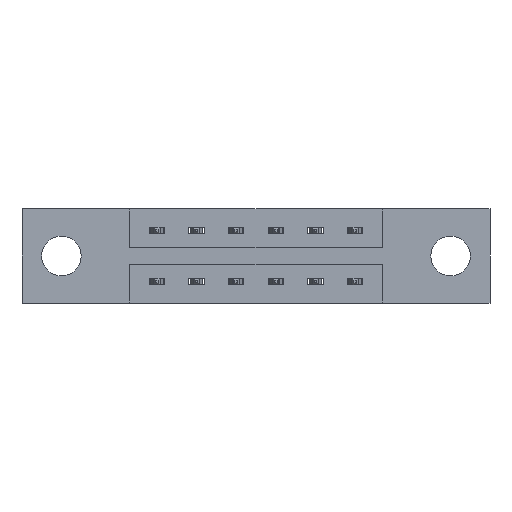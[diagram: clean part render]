
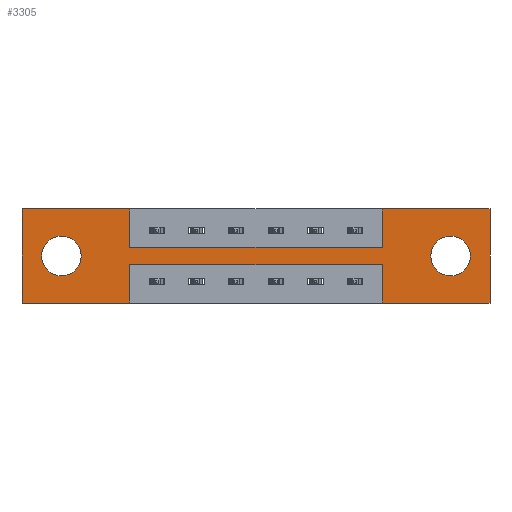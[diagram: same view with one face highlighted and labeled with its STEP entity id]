
A CAD part, front view. The second image highlights one B-rep face of the part: STEP entity #3305.
In plain terms, the highlighted planar face has unit normal (0, -1, 0).
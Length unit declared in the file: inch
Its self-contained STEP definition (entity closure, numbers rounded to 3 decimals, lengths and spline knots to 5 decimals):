
#47 = CARTESIAN_POINT ( 'NONE',  ( 1.687, 0., -0.185 ) ) ;
#235 = DIRECTION ( 'NONE',  ( -1., 0., 0. ) ) ;
#431 = EDGE_CURVE ( 'NONE', #4005, #830, #7189, .T. ) ;
#466 = CARTESIAN_POINT ( 'NONE',  ( 0.155, 0., -0.263 ) ) ;
#543 = CARTESIAN_POINT ( 'NONE',  ( 1.417, 0., -0.37 ) ) ;
#577 = VERTEX_POINT ( 'NONE', #907 ) ;
#745 = VECTOR ( 'NONE', #1510, 39.37008 ) ;
#830 = VERTEX_POINT ( 'NONE', #466 ) ;
#862 = VERTEX_POINT ( 'NONE', #4191 ) ;
#907 = CARTESIAN_POINT ( 'NONE',  ( 0.425, 0., 0. ) ) ;
#922 = DIRECTION ( 'NONE',  ( 0., 0., 1. ) ) ;
#1040 = VERTEX_POINT ( 'NONE', #5908 ) ;
#1049 = CARTESIAN_POINT ( 'NONE',  ( 0., 0., -0.37 ) ) ;
#1073 = EDGE_CURVE ( 'NONE', #1341, #9198, #2133, .T. ) ;
#1083 = ORIENTED_EDGE ( 'NONE', *, *, #4358, .F. ) ;
#1180 = ORIENTED_EDGE ( 'NONE', *, *, #1247, .F. ) ;
#1247 = EDGE_CURVE ( 'NONE', #3250, #5492, #5763, .T. ) ;
#1341 = VERTEX_POINT ( 'NONE', #8503 ) ;
#1447 = LINE ( 'NONE', #6530, #8749 ) ;
#1510 = DIRECTION ( 'NONE',  ( 1., 0., 0. ) ) ;
#1585 = EDGE_CURVE ( 'NONE', #2117, #1040, #1447, .T. ) ;
#1693 = VECTOR ( 'NONE', #5620, 39.37008 ) ;
#1878 = FACE_OUTER_BOUND ( 'NONE', #6573, .T. ) ;
#1929 = VERTEX_POINT ( 'NONE', #9312 ) ;
#1952 = ORIENTED_EDGE ( 'NONE', *, *, #7952, .F. ) ;
#1986 = EDGE_CURVE ( 'NONE', #830, #4005, #7102, .T. ) ;
#2022 = LINE ( 'NONE', #1049, #2926 ) ;
#2030 = EDGE_CURVE ( 'NONE', #862, #2117, #3472, .T. ) ;
#2117 = VERTEX_POINT ( 'NONE', #3014 ) ;
#2133 = LINE ( 'NONE', #7077, #6786 ) ;
#2157 = LINE ( 'NONE', #543, #1693 ) ;
#2166 = CIRCLE ( 'NONE', #7641, 0.078 ) ;
#2237 = ORIENTED_EDGE ( 'NONE', *, *, #8538, .F. ) ;
#2596 = CIRCLE ( 'NONE', #6301, 0.078 ) ;
#2604 = DIRECTION ( 'NONE',  ( 1., 0., 0. ) ) ;
#2738 = CARTESIAN_POINT ( 'NONE',  ( 0.425, 0., -0.37 ) ) ;
#2747 = DIRECTION ( 'NONE',  ( 0., 0., -1. ) ) ;
#2926 = VECTOR ( 'NONE', #6878, 39.37008 ) ;
#2952 = ORIENTED_EDGE ( 'NONE', *, *, #431, .T. ) ;
#3014 = CARTESIAN_POINT ( 'NONE',  ( 1.842, 0., 0. ) ) ;
#3047 = VECTOR ( 'NONE', #922, 39.37008 ) ;
#3053 = ORIENTED_EDGE ( 'NONE', *, *, #2030, .F. ) ;
#3102 = ORIENTED_EDGE ( 'NONE', *, *, #1585, .F. ) ;
#3115 = CARTESIAN_POINT ( 'NONE',  ( 0.425, 0., -0.22 ) ) ;
#3155 = ORIENTED_EDGE ( 'NONE', *, *, #7342, .F. ) ;
#3250 = VERTEX_POINT ( 'NONE', #7258 ) ;
#3305 = ADVANCED_FACE ( 'NONE', ( #5178, #3462, #1878 ), #5323, .T. ) ;
#3322 = VERTEX_POINT ( 'NONE', #4241 ) ;
#3446 = AXIS2_PLACEMENT_3D ( 'NONE', #6985, #6434, #3898 ) ;
#3462 = FACE_BOUND ( 'NONE', #4546, .T. ) ;
#3472 = LINE ( 'NONE', #5888, #745 ) ;
#3476 = CARTESIAN_POINT ( 'NONE',  ( 0., 0., -0.37 ) ) ;
#3681 = ORIENTED_EDGE ( 'NONE', *, *, #6528, .F. ) ;
#3729 = DIRECTION ( 'NONE',  ( 0., 1., 0. ) ) ;
#3753 = EDGE_LOOP ( 'NONE', ( #5044, #5162 ) ) ;
#3898 = DIRECTION ( 'NONE',  ( 0., 0., -1. ) ) ;
#4005 = VERTEX_POINT ( 'NONE', #7033 ) ;
#4191 = CARTESIAN_POINT ( 'NONE',  ( 1.417, 0., 0. ) ) ;
#4241 = CARTESIAN_POINT ( 'NONE',  ( 1.417, 0., -0.22 ) ) ;
#4350 = DIRECTION ( 'NONE',  ( 0., 0., 1. ) ) ;
#4354 = DIRECTION ( 'NONE',  ( 0., 0., 1. ) ) ;
#4358 = EDGE_CURVE ( 'NONE', #3322, #1929, #8828, .T. ) ;
#4497 = CARTESIAN_POINT ( 'NONE',  ( 1.417, 0., -0.15 ) ) ;
#4522 = VERTEX_POINT ( 'NONE', #5004 ) ;
#4546 = EDGE_LOOP ( 'NONE', ( #2952, #4899 ) ) ;
#4674 = LINE ( 'NONE', #8755, #6936 ) ;
#4751 = CARTESIAN_POINT ( 'NONE',  ( 1.417, 0., -0.37 ) ) ;
#4873 = VERTEX_POINT ( 'NONE', #4751 ) ;
#4899 = ORIENTED_EDGE ( 'NONE', *, *, #1986, .T. ) ;
#5004 = CARTESIAN_POINT ( 'NONE',  ( 1.687, 0., -0.107 ) ) ;
#5015 = LINE ( 'NONE', #7655, #3047 ) ;
#5044 = ORIENTED_EDGE ( 'NONE', *, *, #5781, .T. ) ;
#5054 = DIRECTION ( 'NONE',  ( 0., 0., 1. ) ) ;
#5069 = VERTEX_POINT ( 'NONE', #9177 ) ;
#5106 = VECTOR ( 'NONE', #2604, 39.37008 ) ;
#5162 = ORIENTED_EDGE ( 'NONE', *, *, #6592, .T. ) ;
#5178 = FACE_BOUND ( 'NONE', #3753, .T. ) ;
#5182 = DIRECTION ( 'NONE',  ( 0., 0., -1. ) ) ;
#5203 = VECTOR ( 'NONE', #5506, 39.37008 ) ;
#5235 = CARTESIAN_POINT ( 'NONE',  ( 1.687, 0., -0.185 ) ) ;
#5279 = AXIS2_PLACEMENT_3D ( 'NONE', #7938, #8650, #4350 ) ;
#5299 = ORIENTED_EDGE ( 'NONE', *, *, #5520, .F. ) ;
#5323 = PLANE ( 'NONE',  #3446 ) ;
#5492 = VERTEX_POINT ( 'NONE', #4497 ) ;
#5506 = DIRECTION ( 'NONE',  ( 1., 0., 0. ) ) ;
#5520 = EDGE_CURVE ( 'NONE', #1929, #8580, #4674, .T. ) ;
#5620 = DIRECTION ( 'NONE',  ( 0., 0., 1. ) ) ;
#5651 = CARTESIAN_POINT ( 'NONE',  ( 0.425, 0., 0. ) ) ;
#5763 = LINE ( 'NONE', #6945, #5203 ) ;
#5781 = EDGE_CURVE ( 'NONE', #4522, #5069, #2166, .T. ) ;
#5841 = DIRECTION ( 'NONE',  ( 0., 1., 0. ) ) ;
#5888 = CARTESIAN_POINT ( 'NONE',  ( 0., 0., 0. ) ) ;
#5908 = CARTESIAN_POINT ( 'NONE',  ( 1.842, 0., -0.37 ) ) ;
#6062 = AXIS2_PLACEMENT_3D ( 'NONE', #9343, #3729, #5054 ) ;
#6301 = AXIS2_PLACEMENT_3D ( 'NONE', #47, #5841, #8783 ) ;
#6345 = CARTESIAN_POINT ( 'NONE',  ( 0., 0., 0. ) ) ;
#6434 = DIRECTION ( 'NONE',  ( 0., -1., 0. ) ) ;
#6528 = EDGE_CURVE ( 'NONE', #4873, #3322, #2157, .T. ) ;
#6530 = CARTESIAN_POINT ( 'NONE',  ( 1.842, 0., 0. ) ) ;
#6573 = EDGE_LOOP ( 'NONE', ( #5299, #1083, #3681, #3155, #3102, #3053, #1952, #1180, #6626, #8656, #7103, #2237 ) ) ;
#6592 = EDGE_CURVE ( 'NONE', #5069, #4522, #2596, .T. ) ;
#6626 = ORIENTED_EDGE ( 'NONE', *, *, #8055, .F. ) ;
#6692 = VECTOR ( 'NONE', #2747, 39.37008 ) ;
#6729 = DIRECTION ( 'NONE',  ( 0., 0., -1. ) ) ;
#6786 = VECTOR ( 'NONE', #4354, 39.37008 ) ;
#6824 = LINE ( 'NONE', #3476, #7158 ) ;
#6878 = DIRECTION ( 'NONE',  ( -1., 0., 0. ) ) ;
#6936 = VECTOR ( 'NONE', #5182, 39.37008 ) ;
#6945 = CARTESIAN_POINT ( 'NONE',  ( 0.425, 0., -0.15 ) ) ;
#6985 = CARTESIAN_POINT ( 'NONE',  ( 0., 0., -0.37 ) ) ;
#7033 = CARTESIAN_POINT ( 'NONE',  ( 0.155, 0., -0.107 ) ) ;
#7077 = CARTESIAN_POINT ( 'NONE',  ( 0., 0., 0. ) ) ;
#7102 = CIRCLE ( 'NONE', #5279, 0.078 ) ;
#7103 = ORIENTED_EDGE ( 'NONE', *, *, #1073, .F. ) ;
#7158 = VECTOR ( 'NONE', #7818, 39.37008 ) ;
#7189 = CIRCLE ( 'NONE', #6062, 0.078 ) ;
#7247 = DIRECTION ( 'NONE',  ( 0., 0., -1. ) ) ;
#7258 = CARTESIAN_POINT ( 'NONE',  ( 0.425, 0., -0.15 ) ) ;
#7342 = EDGE_CURVE ( 'NONE', #1040, #4873, #6824, .T. ) ;
#7352 = LINE ( 'NONE', #5651, #6692 ) ;
#7641 = AXIS2_PLACEMENT_3D ( 'NONE', #5235, #8060, #6729 ) ;
#7655 = CARTESIAN_POINT ( 'NONE',  ( 1.417, 0., 0. ) ) ;
#7818 = DIRECTION ( 'NONE',  ( -1., 0., 0. ) ) ;
#7938 = CARTESIAN_POINT ( 'NONE',  ( 0.155, 0., -0.185 ) ) ;
#7952 = EDGE_CURVE ( 'NONE', #5492, #862, #5015, .T. ) ;
#8055 = EDGE_CURVE ( 'NONE', #577, #3250, #7352, .T. ) ;
#8060 = DIRECTION ( 'NONE',  ( 0., 1., 0. ) ) ;
#8330 = CARTESIAN_POINT ( 'NONE',  ( 0., 0., 0. ) ) ;
#8373 = EDGE_CURVE ( 'NONE', #9198, #577, #8670, .T. ) ;
#8503 = CARTESIAN_POINT ( 'NONE',  ( 0., 0., -0.37 ) ) ;
#8538 = EDGE_CURVE ( 'NONE', #8580, #1341, #2022, .T. ) ;
#8580 = VERTEX_POINT ( 'NONE', #2738 ) ;
#8606 = VECTOR ( 'NONE', #235, 39.37008 ) ;
#8650 = DIRECTION ( 'NONE',  ( 0., 1., 0. ) ) ;
#8656 = ORIENTED_EDGE ( 'NONE', *, *, #8373, .F. ) ;
#8670 = LINE ( 'NONE', #8330, #5106 ) ;
#8749 = VECTOR ( 'NONE', #7247, 39.37008 ) ;
#8755 = CARTESIAN_POINT ( 'NONE',  ( 0.425, 0., -0.37 ) ) ;
#8783 = DIRECTION ( 'NONE',  ( 0., 0., -1. ) ) ;
#8828 = LINE ( 'NONE', #3115, #8606 ) ;
#9177 = CARTESIAN_POINT ( 'NONE',  ( 1.687, 0., -0.263 ) ) ;
#9198 = VERTEX_POINT ( 'NONE', #6345 ) ;
#9312 = CARTESIAN_POINT ( 'NONE',  ( 0.425, 0., -0.22 ) ) ;
#9343 = CARTESIAN_POINT ( 'NONE',  ( 0.155, 0., -0.185 ) ) ;
